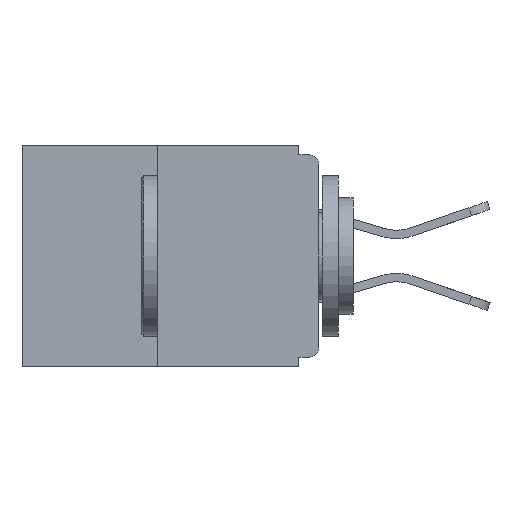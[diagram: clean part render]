
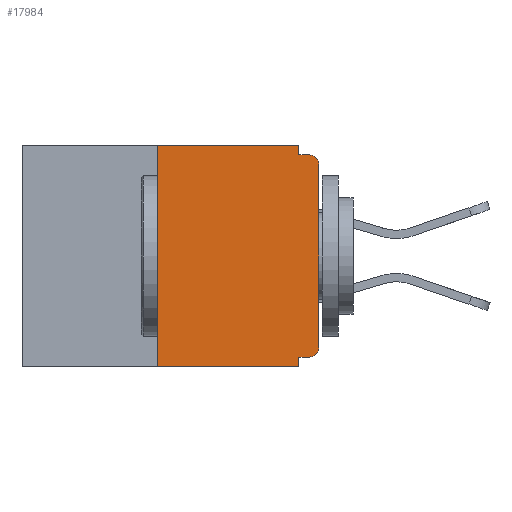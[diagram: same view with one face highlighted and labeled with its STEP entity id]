
A CAD part, left-side view. The second image highlights one B-rep face of the part: STEP entity #17984.
In plain terms, the highlighted planar face has unit normal (-1, 0, 0).
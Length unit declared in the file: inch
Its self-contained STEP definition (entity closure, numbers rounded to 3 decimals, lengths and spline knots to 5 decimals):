
#701 = EDGE_CURVE ( 'NONE', #12387, #14250, #4102, .T. ) ;
#974 = DIRECTION ( 'NONE',  ( 0., 0., -1. ) ) ;
#1000 = VERTEX_POINT ( 'NONE', #16876 ) ;
#1480 = EDGE_CURVE ( 'NONE', #4560, #9554, #7004, .T. ) ;
#1800 = DIRECTION ( 'NONE',  ( 0., 1., 0. ) ) ;
#2089 = VECTOR ( 'NONE', #12219, 39.37008 ) ;
#2441 = VECTOR ( 'NONE', #1800, 39.37008 ) ;
#2544 = CARTESIAN_POINT ( 'NONE',  ( 0., 0.46, 0. ) ) ;
#2711 = DIRECTION ( 'NONE',  ( -1., 0., 0. ) ) ;
#3222 = CIRCLE ( 'NONE', #5871, 0.015 ) ;
#3687 = LINE ( 'NONE', #17277, #14257 ) ;
#4102 = LINE ( 'NONE', #7369, #7778 ) ;
#4318 = PLANE ( 'NONE',  #11926 ) ;
#4560 = VERTEX_POINT ( 'NONE', #18273 ) ;
#4843 = DIRECTION ( 'NONE',  ( 0., 0., 1. ) ) ;
#4846 = FACE_OUTER_BOUND ( 'NONE', #6625, .T. ) ;
#4893 = VECTOR ( 'NONE', #12856, 39.37008 ) ;
#4896 = CARTESIAN_POINT ( 'NONE',  ( 0., 0., -0.328 ) ) ;
#5336 = ORIENTED_EDGE ( 'NONE', *, *, #11124, .T. ) ;
#5506 = DIRECTION ( 'NONE',  ( 0., -1., 0. ) ) ;
#5531 = EDGE_CURVE ( 'NONE', #9554, #15571, #8115, .T. ) ;
#5806 = ORIENTED_EDGE ( 'NONE', *, *, #10138, .T. ) ;
#5871 = AXIS2_PLACEMENT_3D ( 'NONE', #11262, #7898, #12850 ) ;
#5948 = DIRECTION ( 'NONE',  ( 0., 0., -1. ) ) ;
#6083 = CIRCLE ( 'NONE', #8857, 0.015 ) ;
#6396 = ORIENTED_EDGE ( 'NONE', *, *, #10551, .F. ) ;
#6575 = LINE ( 'NONE', #2544, #18557 ) ;
#6625 = EDGE_LOOP ( 'NONE', ( #17426, #7489, #10718, #6396, #9231, #5806, #5336, #9336, #16520, #19018 ) ) ;
#7004 = LINE ( 'NONE', #13669, #2089 ) ;
#7369 = CARTESIAN_POINT ( 'NONE',  ( 0., 0.25, 0. ) ) ;
#7489 = ORIENTED_EDGE ( 'NONE', *, *, #701, .F. ) ;
#7672 = EDGE_CURVE ( 'NONE', #1000, #15571, #6083, .T. ) ;
#7693 = VERTEX_POINT ( 'NONE', #13780 ) ;
#7778 = VECTOR ( 'NONE', #19864, 39.37008 ) ;
#7898 = DIRECTION ( 'NONE',  ( -1., 0., 0. ) ) ;
#8115 = LINE ( 'NONE', #14903, #13278 ) ;
#8615 = DIRECTION ( 'NONE',  ( 0., -1., 0. ) ) ;
#8630 = LINE ( 'NONE', #13770, #18645 ) ;
#8857 = AXIS2_PLACEMENT_3D ( 'NONE', #19982, #2711, #974 ) ;
#9231 = ORIENTED_EDGE ( 'NONE', *, *, #11314, .F. ) ;
#9336 = ORIENTED_EDGE ( 'NONE', *, *, #7672, .T. ) ;
#9554 = VERTEX_POINT ( 'NONE', #15366 ) ;
#9688 = CARTESIAN_POINT ( 'NONE',  ( 0., 0.25, 0. ) ) ;
#10138 = EDGE_CURVE ( 'NONE', #7693, #17874, #3222, .T. ) ;
#10551 = EDGE_CURVE ( 'NONE', #16998, #15950, #8630, .T. ) ;
#10718 = ORIENTED_EDGE ( 'NONE', *, *, #15829, .T. ) ;
#11124 = EDGE_CURVE ( 'NONE', #17874, #1000, #3687, .T. ) ;
#11262 = CARTESIAN_POINT ( 'NONE',  ( 0., 0.015, -0.313 ) ) ;
#11314 = EDGE_CURVE ( 'NONE', #7693, #16998, #18622, .T. ) ;
#11538 = CARTESIAN_POINT ( 'NONE',  ( 0., 0.031, -0.343 ) ) ;
#11926 = AXIS2_PLACEMENT_3D ( 'NONE', #19976, #17031, #18609 ) ;
#12219 = DIRECTION ( 'NONE',  ( 0., 0., -1. ) ) ;
#12387 = VERTEX_POINT ( 'NONE', #17594 ) ;
#12850 = DIRECTION ( 'NONE',  ( 0., 0., -1. ) ) ;
#12856 = DIRECTION ( 'NONE',  ( 0., -1., 0. ) ) ;
#13133 = CARTESIAN_POINT ( 'NONE',  ( 0., 0.031, -0.328 ) ) ;
#13278 = VECTOR ( 'NONE', #8615, 39.37008 ) ;
#13669 = CARTESIAN_POINT ( 'NONE',  ( 0., 0.031, 0. ) ) ;
#13770 = CARTESIAN_POINT ( 'NONE',  ( 0., 0.031, -0.343 ) ) ;
#13780 = CARTESIAN_POINT ( 'NONE',  ( 0., 0.015, -0.328 ) ) ;
#14250 = VERTEX_POINT ( 'NONE', #9688 ) ;
#14257 = VECTOR ( 'NONE', #4843, 39.37008 ) ;
#14903 = CARTESIAN_POINT ( 'NONE',  ( 0., 0., -0.015 ) ) ;
#15366 = CARTESIAN_POINT ( 'NONE',  ( 0., 0.031, -0.015 ) ) ;
#15494 = CARTESIAN_POINT ( 'NONE',  ( 0., 0., -0.313 ) ) ;
#15571 = VERTEX_POINT ( 'NONE', #19865 ) ;
#15829 = EDGE_CURVE ( 'NONE', #12387, #15950, #17888, .T. ) ;
#15950 = VERTEX_POINT ( 'NONE', #11538 ) ;
#16520 = ORIENTED_EDGE ( 'NONE', *, *, #5531, .F. ) ;
#16876 = CARTESIAN_POINT ( 'NONE',  ( 0., 0., -0.03 ) ) ;
#16998 = VERTEX_POINT ( 'NONE', #13133 ) ;
#17031 = DIRECTION ( 'NONE',  ( 1., 0., 0. ) ) ;
#17277 = CARTESIAN_POINT ( 'NONE',  ( 0., 0., 0. ) ) ;
#17426 = ORIENTED_EDGE ( 'NONE', *, *, #17680, .F. ) ;
#17594 = CARTESIAN_POINT ( 'NONE',  ( 0., 0.25, -0.343 ) ) ;
#17680 = EDGE_CURVE ( 'NONE', #14250, #4560, #6575, .T. ) ;
#17874 = VERTEX_POINT ( 'NONE', #15494 ) ;
#17888 = LINE ( 'NONE', #18925, #4893 ) ;
#17984 = ADVANCED_FACE ( 'NONE', ( #4846 ), #4318, .F. ) ;
#18273 = CARTESIAN_POINT ( 'NONE',  ( 0., 0.031, 0. ) ) ;
#18557 = VECTOR ( 'NONE', #5506, 39.37008 ) ;
#18609 = DIRECTION ( 'NONE',  ( 0., 0., -1. ) ) ;
#18622 = LINE ( 'NONE', #4896, #2441 ) ;
#18645 = VECTOR ( 'NONE', #5948, 39.37008 ) ;
#18925 = CARTESIAN_POINT ( 'NONE',  ( 0., 0.46, -0.343 ) ) ;
#19018 = ORIENTED_EDGE ( 'NONE', *, *, #1480, .F. ) ;
#19864 = DIRECTION ( 'NONE',  ( 0., 0., 1. ) ) ;
#19865 = CARTESIAN_POINT ( 'NONE',  ( 0., 0.015, -0.015 ) ) ;
#19976 = CARTESIAN_POINT ( 'NONE',  ( 0., 0.46, 0. ) ) ;
#19982 = CARTESIAN_POINT ( 'NONE',  ( 0., 0.015, -0.03 ) ) ;
